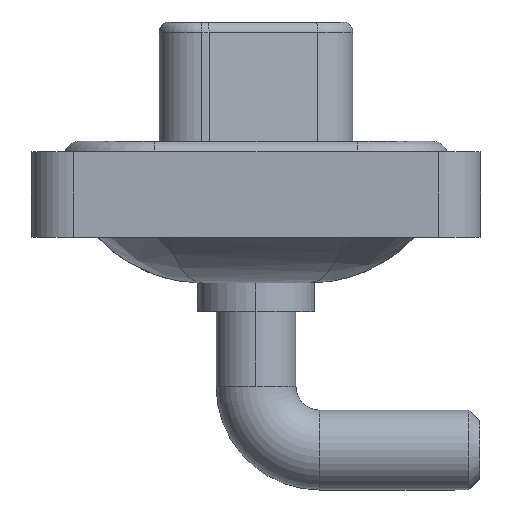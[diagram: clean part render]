
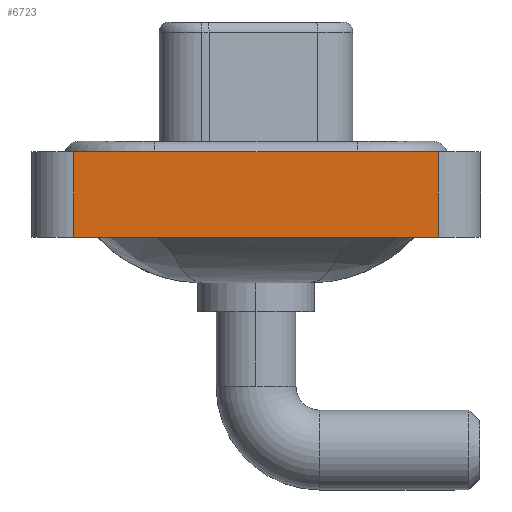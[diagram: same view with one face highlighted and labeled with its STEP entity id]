
A CAD part, left-side view. The second image highlights one B-rep face of the part: STEP entity #6723.
In plain terms, the highlighted planar face has unit normal (-1, 0, 0).
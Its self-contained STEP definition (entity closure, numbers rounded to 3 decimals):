
#141 = FACE_OUTER_BOUND ( 'NONE', #8125, .T. ) ;
#1031 = CARTESIAN_POINT ( 'NONE',  ( -7.25, 8.55, -3.6 ) ) ;
#1332 = EDGE_CURVE ( 'NONE', #6559, #1599, #9891, .T. ) ;
#1520 = VERTEX_POINT ( 'NONE', #1031 ) ;
#1599 = VERTEX_POINT ( 'NONE', #10333 ) ;
#2350 = CARTESIAN_POINT ( 'NONE',  ( -7.25, -8.55, -3.6 ) ) ;
#2605 = CARTESIAN_POINT ( 'NONE',  ( -7.25, 8.55, 0.4 ) ) ;
#3034 = DIRECTION ( 'NONE',  ( 0., 0., 1. ) ) ;
#3618 = ORIENTED_EDGE ( 'NONE', *, *, #1332, .F. ) ;
#4463 = CARTESIAN_POINT ( 'NONE',  ( -7.25, -8.55, 0.4 ) ) ;
#4475 = DIRECTION ( 'NONE',  ( -1., 0., 0. ) ) ;
#4505 = DIRECTION ( 'NONE',  ( 0., 0., 1. ) ) ;
#5197 = EDGE_CURVE ( 'NONE', #1520, #9595, #13371, .T. ) ;
#5747 = DIRECTION ( 'NONE',  ( 0., -1., 0. ) ) ;
#5853 = PLANE ( 'NONE',  #12073 ) ;
#6559 = VERTEX_POINT ( 'NONE', #2605 ) ;
#6723 = ADVANCED_FACE ( 'NONE', ( #141 ), #5853, .T. ) ;
#7191 = CARTESIAN_POINT ( 'NONE',  ( -7.25, 8.55, -3.6 ) ) ;
#7866 = DIRECTION ( 'NONE',  ( 0., -1., 0. ) ) ;
#8125 = EDGE_LOOP ( 'NONE', ( #11024, #3618, #16588, #9914 ) ) ;
#8501 = LINE ( 'NONE', #12644, #17018 ) ;
#8632 = CARTESIAN_POINT ( 'NONE',  ( -7.25, -8.55, -3.6 ) ) ;
#9595 = VERTEX_POINT ( 'NONE', #11803 ) ;
#9709 = LINE ( 'NONE', #7191, #15886 ) ;
#9891 = LINE ( 'NONE', #4463, #16462 ) ;
#9914 = ORIENTED_EDGE ( 'NONE', *, *, #5197, .T. ) ;
#10333 = CARTESIAN_POINT ( 'NONE',  ( -7.25, -8.55, 0.4 ) ) ;
#11024 = ORIENTED_EDGE ( 'NONE', *, *, #14589, .T. ) ;
#11803 = CARTESIAN_POINT ( 'NONE',  ( -7.25, -8.55, -3.6 ) ) ;
#12073 = AXIS2_PLACEMENT_3D ( 'NONE', #8632, #4475, #3034 ) ;
#12596 = DIRECTION ( 'NONE',  ( 0., 0., 1. ) ) ;
#12644 = CARTESIAN_POINT ( 'NONE',  ( -7.25, -8.55, -3.6 ) ) ;
#13371 = LINE ( 'NONE', #2350, #14064 ) ;
#14064 = VECTOR ( 'NONE', #7866, 1000. ) ;
#14589 = EDGE_CURVE ( 'NONE', #9595, #1599, #8501, .T. ) ;
#15511 = EDGE_CURVE ( 'NONE', #1520, #6559, #9709, .T. ) ;
#15886 = VECTOR ( 'NONE', #12596, 1000. ) ;
#16462 = VECTOR ( 'NONE', #5747, 1000. ) ;
#16588 = ORIENTED_EDGE ( 'NONE', *, *, #15511, .F. ) ;
#17018 = VECTOR ( 'NONE', #4505, 1000. ) ;
